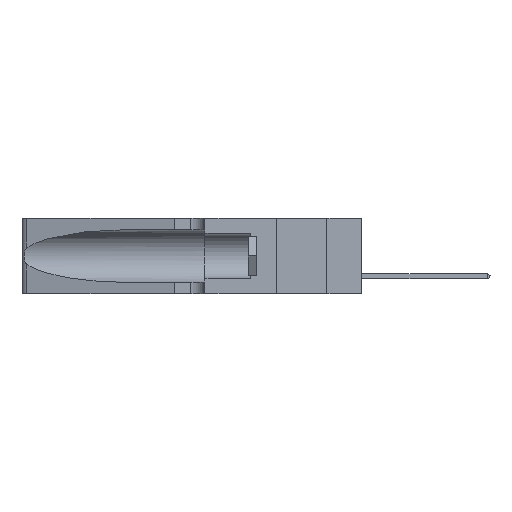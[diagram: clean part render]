
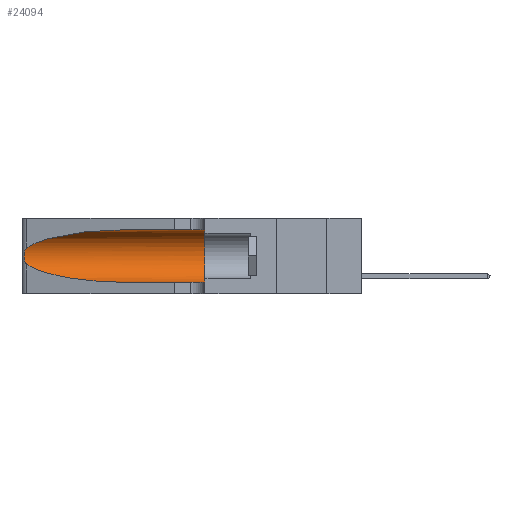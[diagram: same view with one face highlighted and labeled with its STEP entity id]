
A CAD part, left-side view. The second image highlights one B-rep face of the part: STEP entity #24094.
In plain terms, the highlighted cylindrical face has radius 3.308 mm (diameter 6.617 mm), a partial arc.
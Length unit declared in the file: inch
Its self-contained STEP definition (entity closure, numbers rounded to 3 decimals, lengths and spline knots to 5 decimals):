
#994 = CARTESIAN_POINT ( 'NONE',  ( 0.26018, 1.23835, 0.19895 ) ) ;
#1513 = CARTESIAN_POINT ( 'NONE',  ( 0.1305, 0.72297, 0.05475 ) ) ;
#2843 = CARTESIAN_POINT ( 'NONE',  ( 0.1305, 1.61858, 0.31525 ) ) ;
#3802 = B_SPLINE_CURVE_WITH_KNOTS ( 'NONE', 3,
 ( #5440, #18488, #25062, #30357, #27862, #994, #5287, #39089, #37971, #20301, #8672, #4511, #28700, #8661 ),
 .UNSPECIFIED., .F., .F.,
 ( 4, 2, 2, 2, 2, 2, 4 ),
 ( 0., 0.00027, 0.00053, 0.00107, 0.0016, 0.00187, 0.00214 ),
 .UNSPECIFIED. ) ;
#4511 = CARTESIAN_POINT ( 'NONE',  ( 0.25639, 1.23186, 0.15144 ) ) ;
#5287 = CARTESIAN_POINT ( 'NONE',  ( 0.26075, 1.23896, 0.19203 ) ) ;
#5440 = CARTESIAN_POINT ( 'NONE',  ( 0.25487, 1.22718, 0.22369 ) ) ;
#5489 = DIRECTION ( 'NONE',  ( 0., 1., 0. ) ) ;
#5929 = CARTESIAN_POINT ( 'NONE',  ( 0.25487, 1.22718, 0.14631 ) ) ;
#6123 = VERTEX_POINT ( 'NONE', #5929 ) ;
#6908 = VECTOR ( 'NONE', #20252, 39.37008 ) ;
#7860 = DIRECTION ( 'NONE',  ( 0., -1., 0. ) ) ;
#8008 = CARTESIAN_POINT ( 'NONE',  ( 0.1305, 1.61858, 0.185 ) ) ;
#8661 = CARTESIAN_POINT ( 'NONE',  ( 0.25487, 1.22718, 0.14631 ) ) ;
#8672 = CARTESIAN_POINT ( 'NONE',  ( 0.25789, 1.23486, 0.15765 ) ) ;
#8921 = EDGE_CURVE ( 'NONE', #13235, #6123, #3802, .T. ) ;
#8930 = LINE ( 'NONE', #26560, #6908 ) ;
#9100 = CARTESIAN_POINT ( 'NONE',  ( 0.1305, 0.35, 0.31525 ) ) ;
#9941 = ORIENTED_EDGE ( 'NONE', *, *, #16207, .F. ) ;
#10922 =( BOUNDED_CURVE ( )  B_SPLINE_CURVE ( 3, ( #34456, #31269, #24830, #14856 ),
 .UNSPECIFIED., .F., .F. ) 
 B_SPLINE_CURVE_WITH_KNOTS ( ( 4, 4 ),
 ( 3.44316, 4.71239 ),
 .UNSPECIFIED. ) 
 CURVE ( )  GEOMETRIC_REPRESENTATION_ITEM ( )  RATIONAL_B_SPLINE_CURVE ( ( 1., 0.87, 0.87, 1. ) ) 
 REPRESENTATION_ITEM ( '' )  );
#11461 = AXIS2_PLACEMENT_3D ( 'NONE', #8008, #7860, #40857 ) ;
#11751 = CARTESIAN_POINT ( 'NONE',  ( 0.1305, 0.72297, 0.31525 ) ) ;
#12022 = CARTESIAN_POINT ( 'NONE',  ( 0.2373, 1.15595, 0.28018 ) ) ;
#12756 =( BOUNDED_CURVE ( )  B_SPLINE_CURVE ( 3, ( #11751, #25022, #12022, #31625 ),
 .UNSPECIFIED., .F., .F. ) 
 B_SPLINE_CURVE_WITH_KNOTS ( ( 4, 4 ),
 ( 1.5708, 2.84003 ),
 .UNSPECIFIED. ) 
 CURVE ( )  GEOMETRIC_REPRESENTATION_ITEM ( )  RATIONAL_B_SPLINE_CURVE ( ( 1., 0.87, 0.87, 1. ) ) 
 REPRESENTATION_ITEM ( '' )  );
#12840 = VERTEX_POINT ( 'NONE', #9100 ) ;
#13235 = VERTEX_POINT ( 'NONE', #26419 ) ;
#13640 = ORIENTED_EDGE ( 'NONE', *, *, #26647, .F. ) ;
#14034 = ORIENTED_EDGE ( 'NONE', *, *, #8921, .T. ) ;
#14412 = VERTEX_POINT ( 'NONE', #1513 ) ;
#14856 = CARTESIAN_POINT ( 'NONE',  ( 0.1305, 0.72297, 0.05475 ) ) ;
#15843 = ORIENTED_EDGE ( 'NONE', *, *, #32697, .T. ) ;
#15992 = CARTESIAN_POINT ( 'NONE',  ( 0.1305, 0.72297, 0.31525 ) ) ;
#16207 = EDGE_CURVE ( 'NONE', #39922, #12840, #36561, .T. ) ;
#17457 = CYLINDRICAL_SURFACE ( 'NONE', #11461, 0.13025 ) ;
#18488 = CARTESIAN_POINT ( 'NONE',  ( 0.25555, 1.22994, 0.2215 ) ) ;
#19029 = EDGE_CURVE ( 'NONE', #14412, #30359, #8930, .T. ) ;
#20252 = DIRECTION ( 'NONE',  ( 0., -1., 0. ) ) ;
#20301 = CARTESIAN_POINT ( 'NONE',  ( 0.25856, 1.23593, 0.16098 ) ) ;
#24094 = ADVANCED_FACE ( 'NONE', ( #30746 ), #17457, .F. ) ;
#24714 = ORIENTED_EDGE ( 'NONE', *, *, #40973, .T. ) ;
#24830 = CARTESIAN_POINT ( 'NONE',  ( 0.18966, 0.96281, 0.05475 ) ) ;
#24839 = CARTESIAN_POINT ( 'NONE',  ( 0.1305, 0.35, 0.185 ) ) ;
#25022 = CARTESIAN_POINT ( 'NONE',  ( 0.18966, 0.96281, 0.31525 ) ) ;
#25062 = CARTESIAN_POINT ( 'NONE',  ( 0.25639, 1.23184, 0.21858 ) ) ;
#26419 = CARTESIAN_POINT ( 'NONE',  ( 0.25487, 1.22718, 0.22369 ) ) ;
#26560 = CARTESIAN_POINT ( 'NONE',  ( 0.1305, 1.61858, 0.05475 ) ) ;
#26647 = EDGE_CURVE ( 'NONE', #12840, #30359, #27969, .T. ) ;
#27745 = CARTESIAN_POINT ( 'NONE',  ( 0.1305, 0.35, 0.05475 ) ) ;
#27862 = CARTESIAN_POINT ( 'NONE',  ( 0.25854, 1.2359, 0.20912 ) ) ;
#27969 = CIRCLE ( 'NONE', #40932, 0.13025 ) ;
#28311 = EDGE_LOOP ( 'NONE', ( #24714, #14034, #15843, #31726, #13640, #9941 ) ) ;
#28700 = CARTESIAN_POINT ( 'NONE',  ( 0.25555, 1.22993, 0.14849 ) ) ;
#30357 = CARTESIAN_POINT ( 'NONE',  ( 0.25787, 1.23484, 0.2124 ) ) ;
#30359 = VERTEX_POINT ( 'NONE', #27745 ) ;
#30746 = FACE_OUTER_BOUND ( 'NONE', #28311, .T. ) ;
#31269 = CARTESIAN_POINT ( 'NONE',  ( 0.2373, 1.15595, 0.08982 ) ) ;
#31428 = DIRECTION ( 'NONE',  ( 0., 0., 1. ) ) ;
#31625 = CARTESIAN_POINT ( 'NONE',  ( 0.25487, 1.22718, 0.22369 ) ) ;
#31726 = ORIENTED_EDGE ( 'NONE', *, *, #19029, .T. ) ;
#32697 = EDGE_CURVE ( 'NONE', #6123, #14412, #10922, .T. ) ;
#34078 = DIRECTION ( 'NONE',  ( 0., -1., 0. ) ) ;
#34456 = CARTESIAN_POINT ( 'NONE',  ( 0.25487, 1.22718, 0.14631 ) ) ;
#36561 = LINE ( 'NONE', #2843, #40146 ) ;
#37971 = CARTESIAN_POINT ( 'NONE',  ( 0.26017, 1.23833, 0.17102 ) ) ;
#39089 = CARTESIAN_POINT ( 'NONE',  ( 0.26075, 1.23896, 0.178 ) ) ;
#39922 = VERTEX_POINT ( 'NONE', #15992 ) ;
#40146 = VECTOR ( 'NONE', #34078, 39.37008 ) ;
#40857 = DIRECTION ( 'NONE',  ( 0., 0., -1. ) ) ;
#40932 = AXIS2_PLACEMENT_3D ( 'NONE', #24839, #5489, #31428 ) ;
#40973 = EDGE_CURVE ( 'NONE', #39922, #13235, #12756, .T. ) ;
